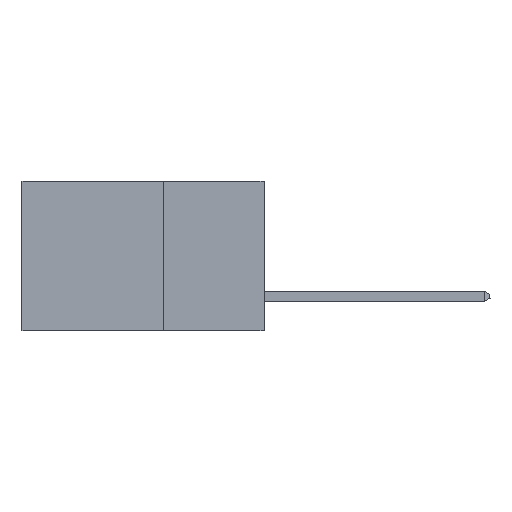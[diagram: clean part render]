
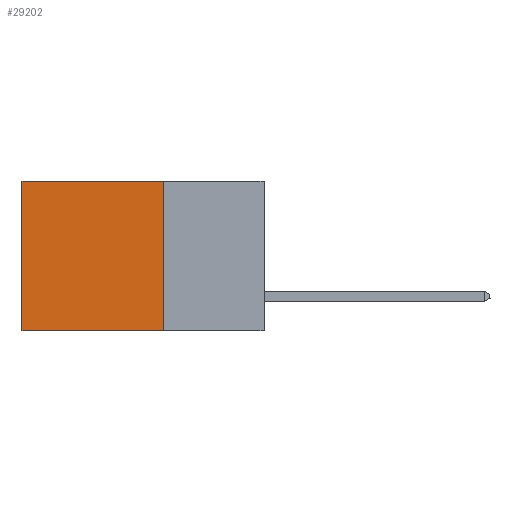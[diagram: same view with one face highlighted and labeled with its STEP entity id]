
A CAD part, left-side view. The second image highlights one B-rep face of the part: STEP entity #29202.
In plain terms, the highlighted planar face has unit normal (-1, 0, 0).
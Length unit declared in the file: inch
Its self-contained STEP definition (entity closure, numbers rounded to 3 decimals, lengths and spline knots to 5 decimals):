
#288 = CARTESIAN_POINT ( 'NONE',  ( 0.298, 0.6, 0. ) ) ;
#1727 = VERTEX_POINT ( 'NONE', #22901 ) ;
#2346 = CARTESIAN_POINT ( 'NONE',  ( 0.298, 0.6, -0.37 ) ) ;
#2842 = LINE ( 'NONE', #288, #20594 ) ;
#3413 = CARTESIAN_POINT ( 'NONE',  ( 0.298, 0.25, 0. ) ) ;
#4011 = VERTEX_POINT ( 'NONE', #14687 ) ;
#4429 = CARTESIAN_POINT ( 'NONE',  ( 0.298, 0.25, 0. ) ) ;
#4508 = EDGE_LOOP ( 'NONE', ( #5656, #5799, #11585, #23198 ) ) ;
#5284 = EDGE_CURVE ( 'NONE', #12956, #4011, #24444, .T. ) ;
#5347 = DIRECTION ( 'NONE',  ( 0., 0., -1. ) ) ;
#5398 = FACE_OUTER_BOUND ( 'NONE', #4508, .T. ) ;
#5538 = PLANE ( 'NONE',  #19597 ) ;
#5656 = ORIENTED_EDGE ( 'NONE', *, *, #15885, .T. ) ;
#5799 = ORIENTED_EDGE ( 'NONE', *, *, #23539, .F. ) ;
#7492 = DIRECTION ( 'NONE',  ( 0., 0., -1. ) ) ;
#10682 = VECTOR ( 'NONE', #24573, 39.37008 ) ;
#11427 = VECTOR ( 'NONE', #29969, 39.37008 ) ;
#11585 = ORIENTED_EDGE ( 'NONE', *, *, #5284, .F. ) ;
#12956 = VERTEX_POINT ( 'NONE', #24145 ) ;
#14538 = CARTESIAN_POINT ( 'NONE',  ( 0.298, 0.25, 0. ) ) ;
#14687 = CARTESIAN_POINT ( 'NONE',  ( 0.298, 0.25, -0.37 ) ) ;
#15789 = LINE ( 'NONE', #18431, #11427 ) ;
#15885 = EDGE_CURVE ( 'NONE', #1727, #23412, #2842, .T. ) ;
#17586 = EDGE_CURVE ( 'NONE', #12956, #1727, #25906, .T. ) ;
#18278 = VECTOR ( 'NONE', #25328, 39.37008 ) ;
#18431 = CARTESIAN_POINT ( 'NONE',  ( 0.298, 0.25, -0.37 ) ) ;
#19597 = AXIS2_PLACEMENT_3D ( 'NONE', #3413, #21747, #5347 ) ;
#20594 = VECTOR ( 'NONE', #7492, 39.37008 ) ;
#21747 = DIRECTION ( 'NONE',  ( 1., 0., 0. ) ) ;
#22901 = CARTESIAN_POINT ( 'NONE',  ( 0.298, 0.6, 0. ) ) ;
#23198 = ORIENTED_EDGE ( 'NONE', *, *, #17586, .T. ) ;
#23412 = VERTEX_POINT ( 'NONE', #2346 ) ;
#23539 = EDGE_CURVE ( 'NONE', #4011, #23412, #15789, .T. ) ;
#24145 = CARTESIAN_POINT ( 'NONE',  ( 0.298, 0.25, 0. ) ) ;
#24444 = LINE ( 'NONE', #4429, #18278 ) ;
#24573 = DIRECTION ( 'NONE',  ( 0., 1., 0. ) ) ;
#25328 = DIRECTION ( 'NONE',  ( 0., 0., -1. ) ) ;
#25906 = LINE ( 'NONE', #14538, #10682 ) ;
#29202 = ADVANCED_FACE ( 'NONE', ( #5398 ), #5538, .F. ) ;
#29969 = DIRECTION ( 'NONE',  ( 0., 1., 0. ) ) ;
